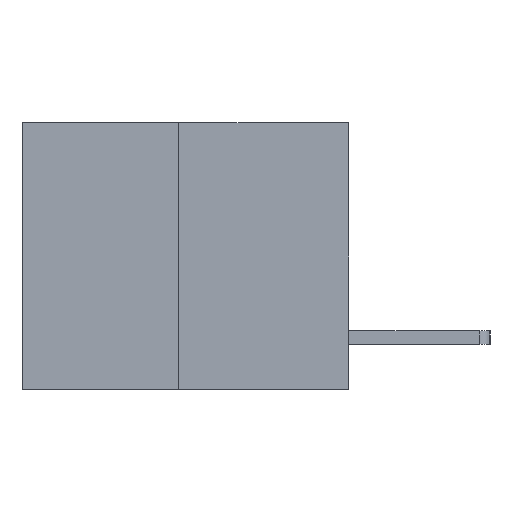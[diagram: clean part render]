
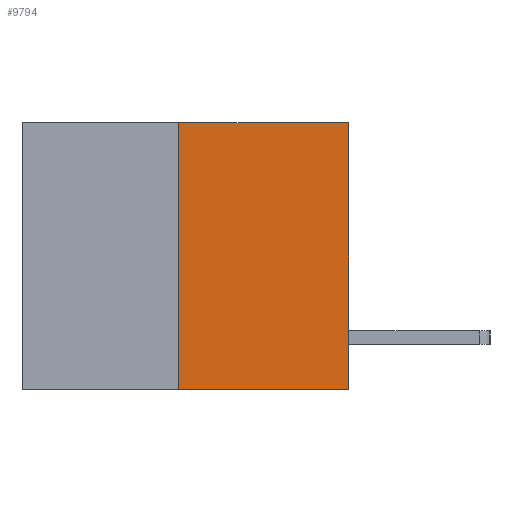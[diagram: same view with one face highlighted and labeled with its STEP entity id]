
A CAD part, left-side view. The second image highlights one B-rep face of the part: STEP entity #9794.
In plain terms, the highlighted planar face has unit normal (-1, 0, 0).
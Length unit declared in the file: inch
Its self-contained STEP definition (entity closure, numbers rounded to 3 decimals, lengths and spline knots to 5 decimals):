
#60 = DIRECTION ( 'NONE',  ( 0., 0., 1. ) ) ;
#263 = ORIENTED_EDGE ( 'NONE', *, *, #8919, .T. ) ;
#364 = EDGE_CURVE ( 'NONE', #4686, #5932, #9200, .T. ) ;
#568 = PLANE ( 'NONE',  #4994 ) ;
#743 = CARTESIAN_POINT ( 'NONE',  ( 0., 0., 0. ) ) ;
#1448 = CARTESIAN_POINT ( 'NONE',  ( 0., 0.6, 0. ) ) ;
#1856 = CARTESIAN_POINT ( 'NONE',  ( 0., 0.312, -0.49 ) ) ;
#2259 = EDGE_LOOP ( 'NONE', ( #8506, #263, #5983, #3082 ) ) ;
#3082 = ORIENTED_EDGE ( 'NONE', *, *, #3242, .F. ) ;
#3225 = VERTEX_POINT ( 'NONE', #743 ) ;
#3242 = EDGE_CURVE ( 'NONE', #5932, #3225, #4928, .T. ) ;
#3812 = CARTESIAN_POINT ( 'NONE',  ( 0., 0., -0.49 ) ) ;
#3951 = CARTESIAN_POINT ( 'NONE',  ( 0., 0., 0. ) ) ;
#4008 = VECTOR ( 'NONE', #60, 39.37008 ) ;
#4113 = CARTESIAN_POINT ( 'NONE',  ( 0., 0.312, 0. ) ) ;
#4316 = DIRECTION ( 'NONE',  ( 1., 0., 0. ) ) ;
#4686 = VERTEX_POINT ( 'NONE', #4908 ) ;
#4829 = DIRECTION ( 'NONE',  ( 0., 0., 1. ) ) ;
#4908 = CARTESIAN_POINT ( 'NONE',  ( 0., 0.312, -0.49 ) ) ;
#4928 = LINE ( 'NONE', #9825, #8157 ) ;
#4994 = AXIS2_PLACEMENT_3D ( 'NONE', #1448, #4316, #9009 ) ;
#5125 = VECTOR ( 'NONE', #4829, 39.37008 ) ;
#5184 = LINE ( 'NONE', #6791, #9512 ) ;
#5273 = DIRECTION ( 'NONE',  ( 0., -1., 0. ) ) ;
#5557 = VERTEX_POINT ( 'NONE', #3812 ) ;
#5932 = VERTEX_POINT ( 'NONE', #4113 ) ;
#5979 = DIRECTION ( 'NONE',  ( 0., -1., 0. ) ) ;
#5983 = ORIENTED_EDGE ( 'NONE', *, *, #9317, .T. ) ;
#6782 = LINE ( 'NONE', #3951, #4008 ) ;
#6791 = CARTESIAN_POINT ( 'NONE',  ( 0., 0.6, -0.49 ) ) ;
#7357 = FACE_OUTER_BOUND ( 'NONE', #2259, .T. ) ;
#8157 = VECTOR ( 'NONE', #5979, 39.37008 ) ;
#8506 = ORIENTED_EDGE ( 'NONE', *, *, #364, .F. ) ;
#8919 = EDGE_CURVE ( 'NONE', #4686, #5557, #5184, .T. ) ;
#9009 = DIRECTION ( 'NONE',  ( 0., 0., -1. ) ) ;
#9200 = LINE ( 'NONE', #1856, #5125 ) ;
#9317 = EDGE_CURVE ( 'NONE', #5557, #3225, #6782, .T. ) ;
#9512 = VECTOR ( 'NONE', #5273, 39.37008 ) ;
#9794 = ADVANCED_FACE ( 'NONE', ( #7357 ), #568, .F. ) ;
#9825 = CARTESIAN_POINT ( 'NONE',  ( 0., 0.6, 0. ) ) ;
